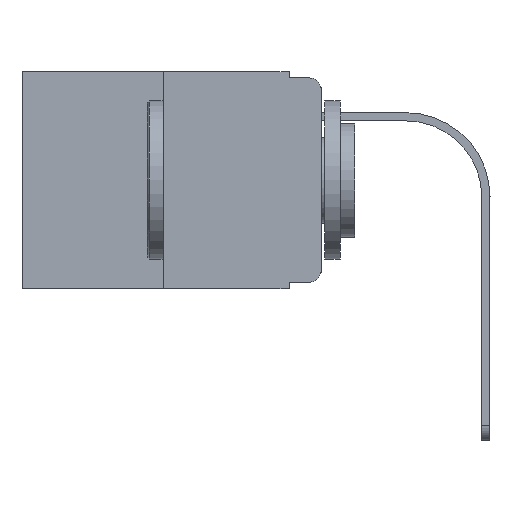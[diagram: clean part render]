
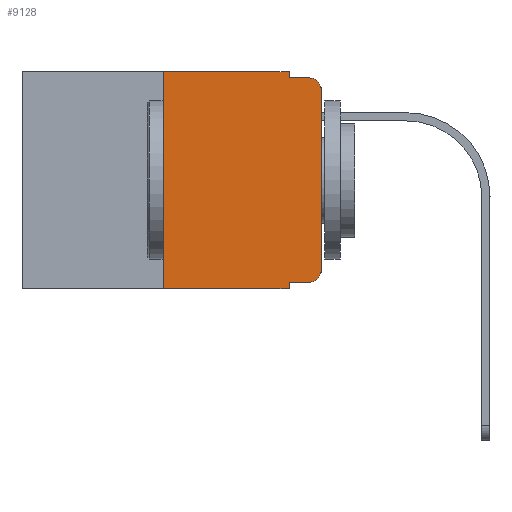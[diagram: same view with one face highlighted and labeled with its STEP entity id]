
A CAD part, left-side view. The second image highlights one B-rep face of the part: STEP entity #9128.
In plain terms, the highlighted planar face has unit normal (-1, 0, 0).
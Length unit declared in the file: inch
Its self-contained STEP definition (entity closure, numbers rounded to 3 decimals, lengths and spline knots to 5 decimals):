
#121 = EDGE_CURVE ( 'NONE', #1371, #8662, #5349, .T. ) ;
#328 = DIRECTION ( 'NONE',  ( -1., 0., 0. ) ) ;
#404 = ORIENTED_EDGE ( 'NONE', *, *, #9778, .F. ) ;
#578 = CIRCLE ( 'NONE', #9218, 0.02 ) ;
#609 = VERTEX_POINT ( 'NONE', #3281 ) ;
#807 = CARTESIAN_POINT ( 'NONE',  ( 0., 0.051, -0.343 ) ) ;
#957 = CARTESIAN_POINT ( 'NONE',  ( 0., 0.473, -0.343 ) ) ;
#1039 = LINE ( 'NONE', #12513, #11632 ) ;
#1044 = EDGE_CURVE ( 'NONE', #1371, #10738, #12759, .T. ) ;
#1347 = CARTESIAN_POINT ( 'NONE',  ( 0., 0.051, 0. ) ) ;
#1371 = VERTEX_POINT ( 'NONE', #8636 ) ;
#1378 = CARTESIAN_POINT ( 'NONE',  ( 0., 0., -0.313 ) ) ;
#1484 = ORIENTED_EDGE ( 'NONE', *, *, #11594, .T. ) ;
#1755 = CARTESIAN_POINT ( 'NONE',  ( 0., 0.02, -0.313 ) ) ;
#1768 = PLANE ( 'NONE',  #8722 ) ;
#1826 = ORIENTED_EDGE ( 'NONE', *, *, #6927, .F. ) ;
#1838 = ORIENTED_EDGE ( 'NONE', *, *, #1044, .T. ) ;
#1862 = CARTESIAN_POINT ( 'NONE',  ( 0., 0.051, -0.01 ) ) ;
#2004 = DIRECTION ( 'NONE',  ( 0., -1., 0. ) ) ;
#2126 = VECTOR ( 'NONE', #7499, 39.37008 ) ;
#2232 = DIRECTION ( 'NONE',  ( 0., 0., 1. ) ) ;
#2579 = VERTEX_POINT ( 'NONE', #1862 ) ;
#2751 = CARTESIAN_POINT ( 'NONE',  ( 0., 0.473, 0. ) ) ;
#3211 = CARTESIAN_POINT ( 'NONE',  ( 0., 0.051, 0. ) ) ;
#3281 = CARTESIAN_POINT ( 'NONE',  ( 0., 0.051, 0. ) ) ;
#3282 = CARTESIAN_POINT ( 'NONE',  ( 0., 0.25, -0.343 ) ) ;
#3639 = LINE ( 'NONE', #7814, #13051 ) ;
#3913 = VERTEX_POINT ( 'NONE', #6435 ) ;
#3991 = DIRECTION ( 'NONE',  ( 1., 0., 0. ) ) ;
#4305 = EDGE_CURVE ( 'NONE', #9912, #5275, #3639, .T. ) ;
#4608 = VERTEX_POINT ( 'NONE', #3282 ) ;
#5073 = LINE ( 'NONE', #6308, #9739 ) ;
#5118 = CARTESIAN_POINT ( 'NONE',  ( 0., 0., -0.03 ) ) ;
#5164 = VECTOR ( 'NONE', #7978, 39.37008 ) ;
#5212 = DIRECTION ( 'NONE',  ( 0., 0., -1. ) ) ;
#5256 = LINE ( 'NONE', #957, #7908 ) ;
#5275 = VERTEX_POINT ( 'NONE', #5118 ) ;
#5332 = CARTESIAN_POINT ( 'NONE',  ( 0., 0.051, -0.333 ) ) ;
#5349 = LINE ( 'NONE', #3211, #12290 ) ;
#5908 = CARTESIAN_POINT ( 'NONE',  ( 0., 0.02, -0.01 ) ) ;
#6166 = EDGE_CURVE ( 'NONE', #2579, #13560, #5073, .T. ) ;
#6308 = CARTESIAN_POINT ( 'NONE',  ( 0., 0.051, -0.01 ) ) ;
#6435 = CARTESIAN_POINT ( 'NONE',  ( 0., 0.25, 0. ) ) ;
#6766 = LINE ( 'NONE', #1347, #7862 ) ;
#6850 = ORIENTED_EDGE ( 'NONE', *, *, #11359, .T. ) ;
#6927 = EDGE_CURVE ( 'NONE', #3913, #609, #12060, .T. ) ;
#7410 = ORIENTED_EDGE ( 'NONE', *, *, #6166, .F. ) ;
#7499 = DIRECTION ( 'NONE',  ( 0., -1., 0. ) ) ;
#7814 = CARTESIAN_POINT ( 'NONE',  ( 0., 0., 0. ) ) ;
#7862 = VECTOR ( 'NONE', #12930, 39.37008 ) ;
#7908 = VECTOR ( 'NONE', #2004, 39.37008 ) ;
#7978 = DIRECTION ( 'NONE',  ( 0., -1., 0. ) ) ;
#8169 = DIRECTION ( 'NONE',  ( 0., 0., -1. ) ) ;
#8243 = FACE_OUTER_BOUND ( 'NONE', #13466, .T. ) ;
#8545 = AXIS2_PLACEMENT_3D ( 'NONE', #1755, #13331, #11481 ) ;
#8636 = CARTESIAN_POINT ( 'NONE',  ( 0., 0.051, -0.333 ) ) ;
#8662 = VERTEX_POINT ( 'NONE', #807 ) ;
#8722 = AXIS2_PLACEMENT_3D ( 'NONE', #2751, #3991, #8169 ) ;
#8725 = CARTESIAN_POINT ( 'NONE',  ( 0., 0.02, -0.03 ) ) ;
#8917 = ORIENTED_EDGE ( 'NONE', *, *, #4305, .T. ) ;
#8980 = EDGE_CURVE ( 'NONE', #609, #2579, #6766, .T. ) ;
#9128 = ADVANCED_FACE ( 'NONE', ( #8243 ), #1768, .F. ) ;
#9218 = AXIS2_PLACEMENT_3D ( 'NONE', #8725, #328, #12952 ) ;
#9739 = VECTOR ( 'NONE', #13670, 39.37008 ) ;
#9778 = EDGE_CURVE ( 'NONE', #4608, #3913, #1039, .T. ) ;
#9796 = CARTESIAN_POINT ( 'NONE',  ( 0., 0.02, -0.333 ) ) ;
#9912 = VERTEX_POINT ( 'NONE', #1378 ) ;
#10307 = ORIENTED_EDGE ( 'NONE', *, *, #10869, .T. ) ;
#10738 = VERTEX_POINT ( 'NONE', #9796 ) ;
#10869 = EDGE_CURVE ( 'NONE', #10738, #9912, #12751, .T. ) ;
#11206 = ORIENTED_EDGE ( 'NONE', *, *, #121, .F. ) ;
#11359 = EDGE_CURVE ( 'NONE', #4608, #8662, #5256, .T. ) ;
#11481 = DIRECTION ( 'NONE',  ( 0., 0., -1. ) ) ;
#11594 = EDGE_CURVE ( 'NONE', #5275, #13560, #578, .T. ) ;
#11632 = VECTOR ( 'NONE', #2232, 39.37008 ) ;
#12060 = LINE ( 'NONE', #12203, #5164 ) ;
#12105 = DIRECTION ( 'NONE',  ( 0., 0., 1. ) ) ;
#12203 = CARTESIAN_POINT ( 'NONE',  ( 0., 0.473, 0. ) ) ;
#12290 = VECTOR ( 'NONE', #5212, 39.37008 ) ;
#12513 = CARTESIAN_POINT ( 'NONE',  ( 0., 0.25, 0. ) ) ;
#12751 = CIRCLE ( 'NONE', #8545, 0.02 ) ;
#12759 = LINE ( 'NONE', #5332, #2126 ) ;
#12930 = DIRECTION ( 'NONE',  ( 0., 0., -1. ) ) ;
#12952 = DIRECTION ( 'NONE',  ( 0., 0., -1. ) ) ;
#13051 = VECTOR ( 'NONE', #12105, 39.37008 ) ;
#13331 = DIRECTION ( 'NONE',  ( -1., 0., 0. ) ) ;
#13402 = ORIENTED_EDGE ( 'NONE', *, *, #8980, .F. ) ;
#13466 = EDGE_LOOP ( 'NONE', ( #8917, #1484, #7410, #13402, #1826, #404, #6850, #11206, #1838, #10307 ) ) ;
#13560 = VERTEX_POINT ( 'NONE', #5908 ) ;
#13670 = DIRECTION ( 'NONE',  ( 0., -1., 0. ) ) ;
